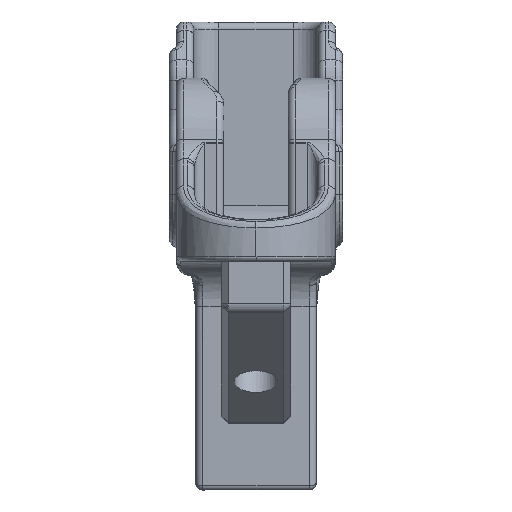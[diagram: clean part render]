
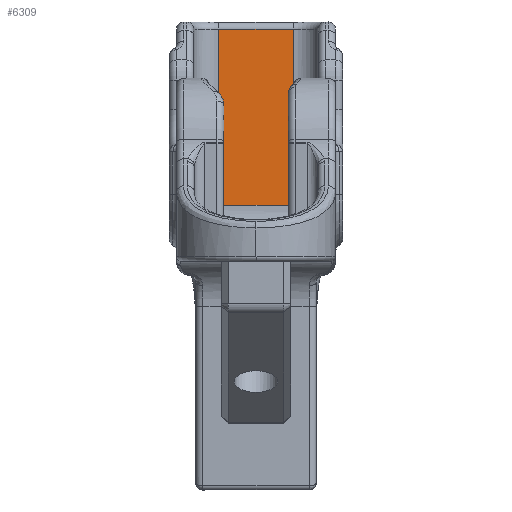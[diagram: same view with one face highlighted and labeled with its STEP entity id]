
A CAD part, left-side view. The second image highlights one B-rep face of the part: STEP entity #6309.
In plain terms, the highlighted planar face has unit normal (-1, 0, 0).
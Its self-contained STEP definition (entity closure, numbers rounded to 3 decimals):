
#326=PLANE('',#6952);
#527=LINE('',#11588,#849);
#528=LINE('',#11601,#850);
#529=LINE('',#11605,#851);
#530=LINE('',#11606,#852);
#849=VECTOR('',#8340,10.);
#850=VECTOR('',#8343,10.);
#851=VECTOR('',#8348,10.);
#852=VECTOR('',#8349,10.);
#1298=FACE_OUTER_BOUND('',#1719,.T.);
#1719=EDGE_LOOP('',(#4820,#4821,#4822,#4823));
#2820=VERTEX_POINT('',#11576);
#2821=VERTEX_POINT('',#11587);
#2822=VERTEX_POINT('',#11600);
#2823=VERTEX_POINT('',#11604);
#3546=EDGE_CURVE('',#2820,#2821,#527,.T.);
#3548=EDGE_CURVE('',#2821,#2822,#528,.T.);
#3550=EDGE_CURVE('',#2820,#2823,#529,.T.);
#3551=EDGE_CURVE('',#2822,#2823,#530,.T.);
#4820=ORIENTED_EDGE('',*,*,#3546,.F.);
#4821=ORIENTED_EDGE('',*,*,#3550,.T.);
#4822=ORIENTED_EDGE('',*,*,#3551,.F.);
#4823=ORIENTED_EDGE('',*,*,#3548,.F.);
#6309=ADVANCED_FACE('',(#1298),#326,.T.);
#6952=AXIS2_PLACEMENT_3D('',#11603,#8346,#8347);
#8340=DIRECTION('',(0.,1.,0.));
#8343=DIRECTION('',(0.,0.,1.));
#8346=DIRECTION('center_axis',(-1.,0.,0.));
#8347=DIRECTION('ref_axis',(0.,1.,0.));
#8348=DIRECTION('',(0.,0.,1.));
#8349=DIRECTION('',(0.,-1.,0.));
#11576=CARTESIAN_POINT('',(-16.793,-5.263,39.998));
#11587=CARTESIAN_POINT('',(-16.793,5.263,39.998));
#11588=CARTESIAN_POINT('',(-16.793,-1.774,39.998));
#11600=CARTESIAN_POINT('',(-16.793,5.263,64.722));
#11601=CARTESIAN_POINT('',(-16.793,5.263,67.175));
#11603=CARTESIAN_POINT('Origin',(-16.793,-3.548,67.175));
#11604=CARTESIAN_POINT('',(-16.793,-5.263,64.723));
#11605=CARTESIAN_POINT('',(-16.793,-5.263,67.175));
#11606=CARTESIAN_POINT('',(-16.793,6.584,64.722));
